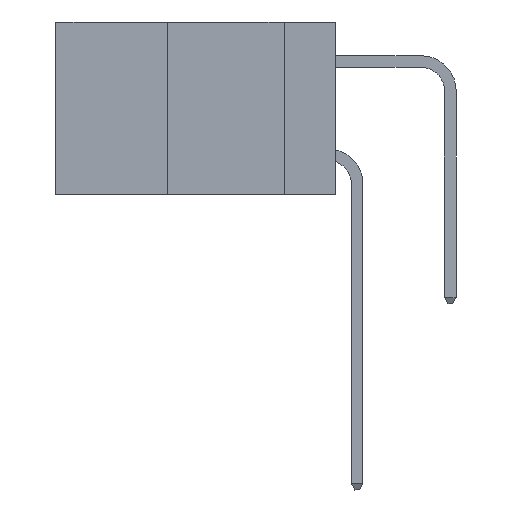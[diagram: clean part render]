
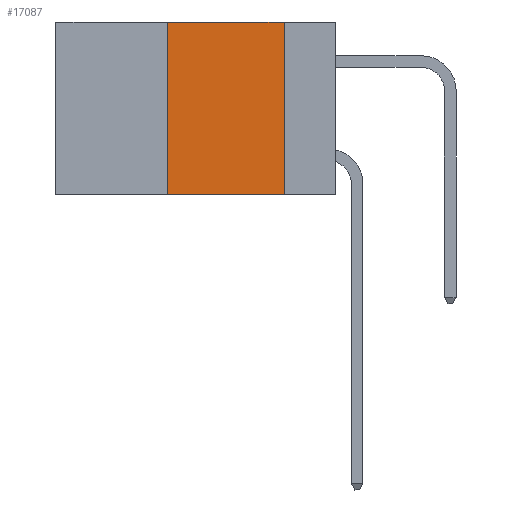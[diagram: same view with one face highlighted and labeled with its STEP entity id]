
A CAD part, left-side view. The second image highlights one B-rep face of the part: STEP entity #17087.
In plain terms, the highlighted planar face has unit normal (-1, 0, 0).
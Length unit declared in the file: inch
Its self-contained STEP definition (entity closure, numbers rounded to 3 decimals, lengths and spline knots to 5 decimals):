
#348 = CARTESIAN_POINT ( 'NONE',  ( 0., 0.11, 0. ) ) ;
#1990 = DIRECTION ( 'NONE',  ( 0., 0., -1. ) ) ;
#2805 = LINE ( 'NONE', #15004, #6480 ) ;
#4092 = LINE ( 'NONE', #348, #15661 ) ;
#4733 = ORIENTED_EDGE ( 'NONE', *, *, #4779, .F. ) ;
#4779 = EDGE_CURVE ( 'NONE', #12882, #12406, #4092, .T. ) ;
#4875 = ORIENTED_EDGE ( 'NONE', *, *, #10011, .F. ) ;
#4953 = ORIENTED_EDGE ( 'NONE', *, *, #5174, .F. ) ;
#5052 = LINE ( 'NONE', #12587, #12188 ) ;
#5056 = PLANE ( 'NONE',  #18384 ) ;
#5073 = ORIENTED_EDGE ( 'NONE', *, *, #18226, .T. ) ;
#5174 = EDGE_CURVE ( 'NONE', #17039, #15260, #16091, .T. ) ;
#5796 = FACE_OUTER_BOUND ( 'NONE', #6169, .T. ) ;
#6169 = EDGE_LOOP ( 'NONE', ( #4733, #4875, #4953, #5073 ) ) ;
#6480 = VECTOR ( 'NONE', #15063, 39.37008 ) ;
#6594 = DIRECTION ( 'NONE',  ( 0., 0., -1. ) ) ;
#8211 = CARTESIAN_POINT ( 'NONE',  ( 0., 0.36, 0. ) ) ;
#9152 = CARTESIAN_POINT ( 'NONE',  ( 0., 0.36, 0. ) ) ;
#10011 = EDGE_CURVE ( 'NONE', #15260, #12882, #2805, .T. ) ;
#10521 = CARTESIAN_POINT ( 'NONE',  ( 0., 0.11, 0. ) ) ;
#11066 = CARTESIAN_POINT ( 'NONE',  ( 0., 0.36, -0.37 ) ) ;
#11093 = DIRECTION ( 'NONE',  ( 0., -1., 0. ) ) ;
#12188 = VECTOR ( 'NONE', #11093, 39.37008 ) ;
#12202 = VECTOR ( 'NONE', #15051, 39.37008 ) ;
#12362 = CARTESIAN_POINT ( 'NONE',  ( 0., 0.11, -0.37 ) ) ;
#12406 = VERTEX_POINT ( 'NONE', #12362 ) ;
#12587 = CARTESIAN_POINT ( 'NONE',  ( 0., 0.6, -0.37 ) ) ;
#12882 = VERTEX_POINT ( 'NONE', #10521 ) ;
#14107 = CARTESIAN_POINT ( 'NONE',  ( 0., 0.6, 0. ) ) ;
#15004 = CARTESIAN_POINT ( 'NONE',  ( 0., 0.6, 0. ) ) ;
#15051 = DIRECTION ( 'NONE',  ( 0., 0., 1. ) ) ;
#15063 = DIRECTION ( 'NONE',  ( 0., -1., 0. ) ) ;
#15260 = VERTEX_POINT ( 'NONE', #8211 ) ;
#15570 = DIRECTION ( 'NONE',  ( 1., 0., 0. ) ) ;
#15661 = VECTOR ( 'NONE', #1990, 39.37008 ) ;
#16091 = LINE ( 'NONE', #9152, #12202 ) ;
#17039 = VERTEX_POINT ( 'NONE', #11066 ) ;
#17087 = ADVANCED_FACE ( 'NONE', ( #5796 ), #5056, .F. ) ;
#18226 = EDGE_CURVE ( 'NONE', #17039, #12406, #5052, .T. ) ;
#18384 = AXIS2_PLACEMENT_3D ( 'NONE', #14107, #15570, #6594 ) ;
